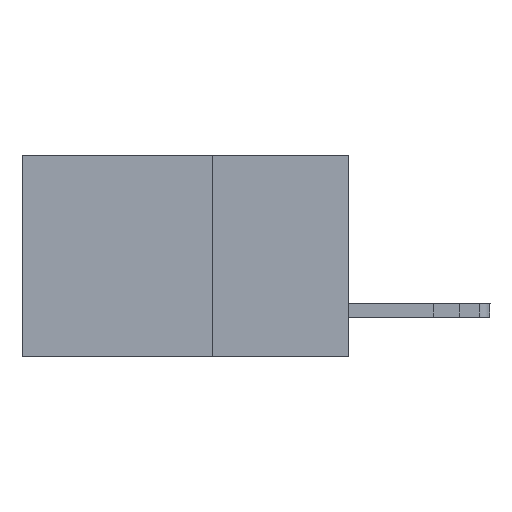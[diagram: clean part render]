
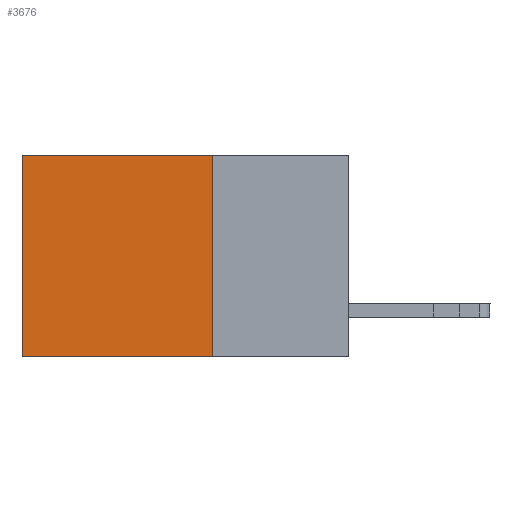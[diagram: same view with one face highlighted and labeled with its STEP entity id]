
A CAD part, left-side view. The second image highlights one B-rep face of the part: STEP entity #3676.
In plain terms, the highlighted planar face has unit normal (-1, 0, 0).
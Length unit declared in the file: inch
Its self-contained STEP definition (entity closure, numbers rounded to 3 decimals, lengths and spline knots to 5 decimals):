
#581 = VERTEX_POINT ( 'NONE', #19948 ) ;
#1379 = CARTESIAN_POINT ( 'NONE',  ( 0.2615, 0.25, 0. ) ) ;
#1923 = CARTESIAN_POINT ( 'NONE',  ( 0.2615, 0.6, -0.37 ) ) ;
#2136 = FACE_OUTER_BOUND ( 'NONE', #5964, .T. ) ;
#3549 = DIRECTION ( 'NONE',  ( 0., 0., -1. ) ) ;
#3622 = ORIENTED_EDGE ( 'NONE', *, *, #19614, .T. ) ;
#3676 = ADVANCED_FACE ( 'NONE', ( #2136 ), #9580, .F. ) ;
#4551 = ORIENTED_EDGE ( 'NONE', *, *, #16372, .F. ) ;
#4939 = CARTESIAN_POINT ( 'NONE',  ( 0.2615, 0.25, -0.37 ) ) ;
#5075 = LINE ( 'NONE', #18314, #9869 ) ;
#5964 = EDGE_LOOP ( 'NONE', ( #3622, #4551, #7522, #6980 ) ) ;
#6162 = LINE ( 'NONE', #9813, #14242 ) ;
#6363 = CARTESIAN_POINT ( 'NONE',  ( 0.2615, 0.25, -0.37 ) ) ;
#6980 = ORIENTED_EDGE ( 'NONE', *, *, #9028, .T. ) ;
#7522 = ORIENTED_EDGE ( 'NONE', *, *, #14371, .F. ) ;
#7566 = CARTESIAN_POINT ( 'NONE',  ( 0.2615, 0.6, 0. ) ) ;
#8611 = DIRECTION ( 'NONE',  ( 0., 0., -1. ) ) ;
#9028 = EDGE_CURVE ( 'NONE', #16458, #17617, #6162, .T. ) ;
#9487 = DIRECTION ( 'NONE',  ( 0., 1., 0. ) ) ;
#9502 = VECTOR ( 'NONE', #3549, 39.37008 ) ;
#9510 = DIRECTION ( 'NONE',  ( 1., 0., 0. ) ) ;
#9580 = PLANE ( 'NONE',  #16384 ) ;
#9655 = DIRECTION ( 'NONE',  ( 0., 0., -1. ) ) ;
#9813 = CARTESIAN_POINT ( 'NONE',  ( 0.2615, 0.25, 0. ) ) ;
#9869 = VECTOR ( 'NONE', #8611, 39.37008 ) ;
#12825 = VECTOR ( 'NONE', #15669, 39.37008 ) ;
#13321 = LINE ( 'NONE', #1923, #9502 ) ;
#13327 = LINE ( 'NONE', #20334, #12825 ) ;
#14242 = VECTOR ( 'NONE', #9487, 39.37008 ) ;
#14371 = EDGE_CURVE ( 'NONE', #16458, #19457, #5075, .T. ) ;
#15669 = DIRECTION ( 'NONE',  ( 0., 1., 0. ) ) ;
#16372 = EDGE_CURVE ( 'NONE', #19457, #581, #13327, .T. ) ;
#16384 = AXIS2_PLACEMENT_3D ( 'NONE', #4939, #9510, #9655 ) ;
#16458 = VERTEX_POINT ( 'NONE', #1379 ) ;
#17617 = VERTEX_POINT ( 'NONE', #7566 ) ;
#18314 = CARTESIAN_POINT ( 'NONE',  ( 0.2615, 0.25, -0.37 ) ) ;
#19457 = VERTEX_POINT ( 'NONE', #6363 ) ;
#19614 = EDGE_CURVE ( 'NONE', #17617, #581, #13321, .T. ) ;
#19948 = CARTESIAN_POINT ( 'NONE',  ( 0.2615, 0.6, -0.37 ) ) ;
#20334 = CARTESIAN_POINT ( 'NONE',  ( 0.2615, 0.25, -0.37 ) ) ;
